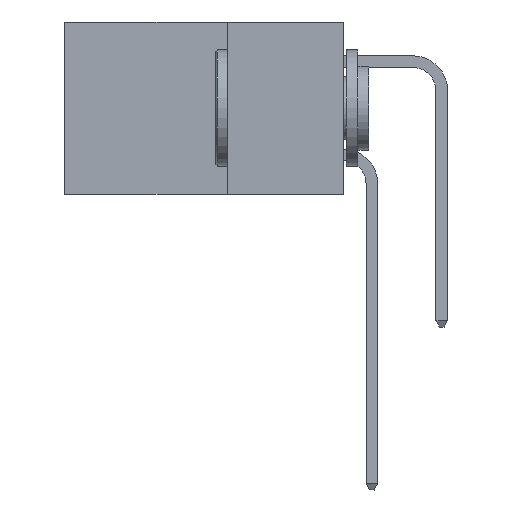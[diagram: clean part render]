
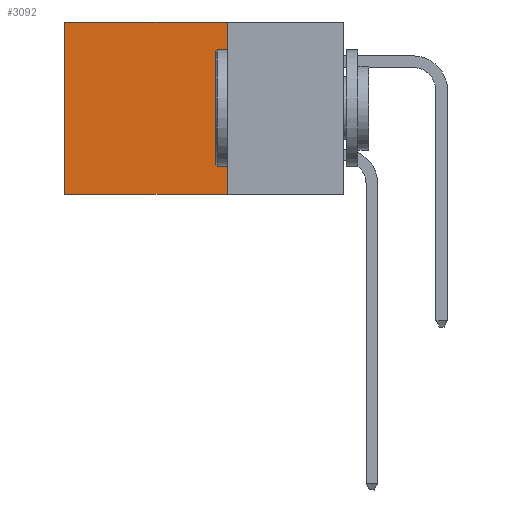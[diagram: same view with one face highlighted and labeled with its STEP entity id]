
A CAD part, left-side view. The second image highlights one B-rep face of the part: STEP entity #3092.
In plain terms, the highlighted planar face has unit normal (-1, 0, 0).
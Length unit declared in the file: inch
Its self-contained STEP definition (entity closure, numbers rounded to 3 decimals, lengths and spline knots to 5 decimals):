
#331 = EDGE_LOOP ( 'NONE', ( #10261, #3930, #17762, #1717 ) ) ;
#1468 = EDGE_CURVE ( 'NONE', #26432, #29685, #18735, .T. ) ;
#1717 = ORIENTED_EDGE ( 'NONE', *, *, #28777, .T. ) ;
#2379 = DIRECTION ( 'NONE',  ( 0., 0., -1. ) ) ;
#2779 = CARTESIAN_POINT ( 'NONE',  ( 0.298, 0.25, 0. ) ) ;
#3092 = ADVANCED_FACE ( 'NONE', ( #6526 ), #17167, .F. ) ;
#3930 = ORIENTED_EDGE ( 'NONE', *, *, #6757, .F. ) ;
#6244 = LINE ( 'NONE', #27855, #7376 ) ;
#6526 = FACE_OUTER_BOUND ( 'NONE', #331, .T. ) ;
#6757 = EDGE_CURVE ( 'NONE', #20695, #29685, #6244, .T. ) ;
#7163 = CARTESIAN_POINT ( 'NONE',  ( 0.298, 0.25, -0.37 ) ) ;
#7376 = VECTOR ( 'NONE', #8648, 39.37008 ) ;
#8422 = DIRECTION ( 'NONE',  ( 0., 0., -1. ) ) ;
#8648 = DIRECTION ( 'NONE',  ( 0., 1., 0. ) ) ;
#9080 = VECTOR ( 'NONE', #8422, 39.37008 ) ;
#10261 = ORIENTED_EDGE ( 'NONE', *, *, #1468, .T. ) ;
#10691 = CARTESIAN_POINT ( 'NONE',  ( 0.298, 0.6, -0.37 ) ) ;
#13021 = CARTESIAN_POINT ( 'NONE',  ( 0.298, 0.25, 0. ) ) ;
#13477 = CARTESIAN_POINT ( 'NONE',  ( 0.298, 0.25, 0. ) ) ;
#14890 = DIRECTION ( 'NONE',  ( 0., 1., 0. ) ) ;
#15457 = AXIS2_PLACEMENT_3D ( 'NONE', #31058, #21752, #2379 ) ;
#16427 = CARTESIAN_POINT ( 'NONE',  ( 0.298, 0.6, 0. ) ) ;
#17167 = PLANE ( 'NONE',  #15457 ) ;
#17762 = ORIENTED_EDGE ( 'NONE', *, *, #22202, .F. ) ;
#18331 = VECTOR ( 'NONE', #21132, 39.37008 ) ;
#18735 = LINE ( 'NONE', #16427, #18331 ) ;
#20695 = VERTEX_POINT ( 'NONE', #7163 ) ;
#21132 = DIRECTION ( 'NONE',  ( 0., 0., -1. ) ) ;
#21752 = DIRECTION ( 'NONE',  ( 1., 0., 0. ) ) ;
#21857 = CARTESIAN_POINT ( 'NONE',  ( 0.298, 0.6, 0. ) ) ;
#21881 = LINE ( 'NONE', #13477, #9080 ) ;
#22202 = EDGE_CURVE ( 'NONE', #30263, #20695, #21881, .T. ) ;
#22218 = LINE ( 'NONE', #2779, #24785 ) ;
#24785 = VECTOR ( 'NONE', #14890, 39.37008 ) ;
#26432 = VERTEX_POINT ( 'NONE', #21857 ) ;
#27855 = CARTESIAN_POINT ( 'NONE',  ( 0.298, 0.25, -0.37 ) ) ;
#28777 = EDGE_CURVE ( 'NONE', #30263, #26432, #22218, .T. ) ;
#29685 = VERTEX_POINT ( 'NONE', #10691 ) ;
#30263 = VERTEX_POINT ( 'NONE', #13021 ) ;
#31058 = CARTESIAN_POINT ( 'NONE',  ( 0.298, 0.25, 0. ) ) ;
